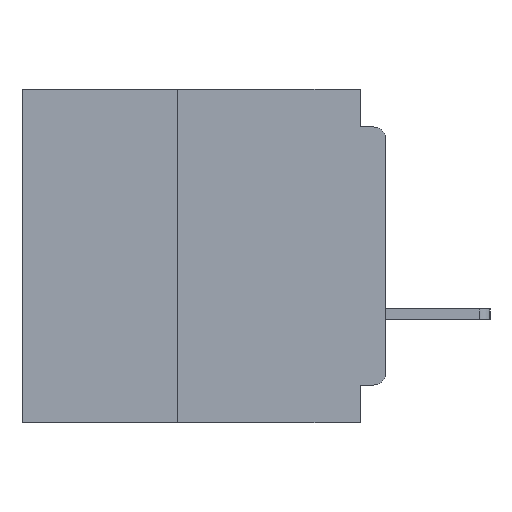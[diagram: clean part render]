
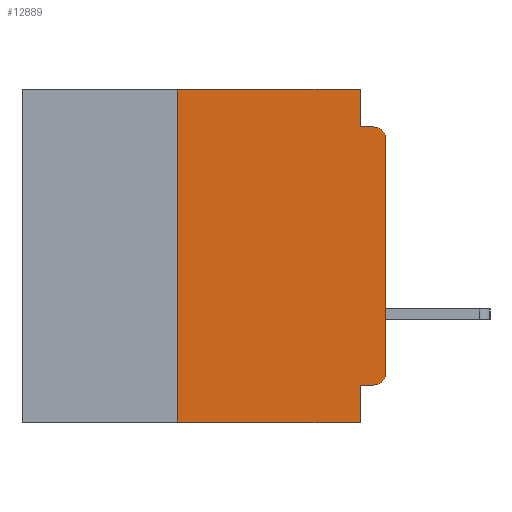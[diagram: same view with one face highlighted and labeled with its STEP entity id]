
A CAD part, left-side view. The second image highlights one B-rep face of the part: STEP entity #12889.
In plain terms, the highlighted planar face has unit normal (-1, 0, 0).
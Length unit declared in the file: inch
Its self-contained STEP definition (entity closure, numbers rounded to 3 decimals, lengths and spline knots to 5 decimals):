
#894 = VECTOR ( 'NONE', #27763, 39.37008 ) ;
#1189 = DIRECTION ( 'NONE',  ( 0., -1., 0. ) ) ;
#1572 = VECTOR ( 'NONE', #20749, 39.37008 ) ;
#1617 = CARTESIAN_POINT ( 'NONE',  ( 0., 0.031, 0. ) ) ;
#1708 = DIRECTION ( 'NONE',  ( 0., 1., 0. ) ) ;
#2461 = LINE ( 'NONE', #29116, #23068 ) ;
#2512 = VERTEX_POINT ( 'NONE', #29915 ) ;
#2609 = VECTOR ( 'NONE', #8462, 39.37008 ) ;
#3530 = CARTESIAN_POINT ( 'NONE',  ( 0., 0.015, -0.355 ) ) ;
#3698 = EDGE_CURVE ( 'NONE', #7731, #6181, #22381, .T. ) ;
#3965 = CARTESIAN_POINT ( 'NONE',  ( 0., 0., -0.045 ) ) ;
#4572 = LINE ( 'NONE', #8036, #33485 ) ;
#5168 = VERTEX_POINT ( 'NONE', #3530 ) ;
#6181 = VERTEX_POINT ( 'NONE', #33322 ) ;
#6646 = DIRECTION ( 'NONE',  ( 0., 0., 1. ) ) ;
#7092 = LINE ( 'NONE', #17834, #35963 ) ;
#7236 = CARTESIAN_POINT ( 'NONE',  ( 0., 0.25, 0. ) ) ;
#7731 = VERTEX_POINT ( 'NONE', #15136 ) ;
#8036 = CARTESIAN_POINT ( 'NONE',  ( 0., 0., 0. ) ) ;
#8047 = VERTEX_POINT ( 'NONE', #27695 ) ;
#8178 = DIRECTION ( 'NONE',  ( 1., 0., 0. ) ) ;
#8462 = DIRECTION ( 'NONE',  ( 0., -1., 0. ) ) ;
#9042 = LINE ( 'NONE', #3965, #1572 ) ;
#9081 = EDGE_CURVE ( 'NONE', #5168, #8047, #14440, .T. ) ;
#9394 = ORIENTED_EDGE ( 'NONE', *, *, #10182, .F. ) ;
#9416 = AXIS2_PLACEMENT_3D ( 'NONE', #24971, #8178, #27771 ) ;
#9592 = ORIENTED_EDGE ( 'NONE', *, *, #22513, .F. ) ;
#10182 = EDGE_CURVE ( 'NONE', #14517, #32678, #2461, .T. ) ;
#10207 = EDGE_CURVE ( 'NONE', #2512, #6181, #9042, .T. ) ;
#10853 = EDGE_CURVE ( 'NONE', #17655, #32678, #15189, .T. ) ;
#11139 = ORIENTED_EDGE ( 'NONE', *, *, #26817, .T. ) ;
#11336 = VERTEX_POINT ( 'NONE', #1617 ) ;
#12762 = CARTESIAN_POINT ( 'NONE',  ( 0., 0.015, -0.34 ) ) ;
#12889 = ADVANCED_FACE ( 'NONE', ( #33016 ), #13725, .F. ) ;
#13714 = CARTESIAN_POINT ( 'NONE',  ( 0., 0.031, 0. ) ) ;
#13725 = PLANE ( 'NONE',  #9416 ) ;
#14182 = ORIENTED_EDGE ( 'NONE', *, *, #3698, .T. ) ;
#14440 = CIRCLE ( 'NONE', #27899, 0.015 ) ;
#14517 = VERTEX_POINT ( 'NONE', #16748 ) ;
#15136 = CARTESIAN_POINT ( 'NONE',  ( 0., 0., -0.06 ) ) ;
#15189 = LINE ( 'NONE', #18070, #30052 ) ;
#15606 = DIRECTION ( 'NONE',  ( 0., 0., -1. ) ) ;
#16748 = CARTESIAN_POINT ( 'NONE',  ( 0., 0.031, -0.355 ) ) ;
#17655 = VERTEX_POINT ( 'NONE', #21581 ) ;
#17820 = ORIENTED_EDGE ( 'NONE', *, *, #25474, .F. ) ;
#17834 = CARTESIAN_POINT ( 'NONE',  ( 0., 0.25, -0.4 ) ) ;
#17948 = ORIENTED_EDGE ( 'NONE', *, *, #18972, .F. ) ;
#17984 = DIRECTION ( 'NONE',  ( 0., 0., -1. ) ) ;
#18070 = CARTESIAN_POINT ( 'NONE',  ( 0., 0.437, -0.4 ) ) ;
#18972 = EDGE_CURVE ( 'NONE', #11336, #2512, #30738, .T. ) ;
#18995 = ORIENTED_EDGE ( 'NONE', *, *, #9081, .T. ) ;
#20749 = DIRECTION ( 'NONE',  ( 0., -1., 0. ) ) ;
#20850 = EDGE_CURVE ( 'NONE', #17655, #29477, #7092, .T. ) ;
#21461 = CARTESIAN_POINT ( 'NONE',  ( 0., 0., -0.355 ) ) ;
#21581 = CARTESIAN_POINT ( 'NONE',  ( 0., 0.25, -0.4 ) ) ;
#22381 = CIRCLE ( 'NONE', #29871, 0.015 ) ;
#22513 = EDGE_CURVE ( 'NONE', #29477, #11336, #24128, .T. ) ;
#22754 = CARTESIAN_POINT ( 'NONE',  ( 0., 0.031, -0.4 ) ) ;
#23068 = VECTOR ( 'NONE', #17984, 39.37008 ) ;
#23440 = ORIENTED_EDGE ( 'NONE', *, *, #10853, .T. ) ;
#23754 = EDGE_LOOP ( 'NONE', ( #11139, #14182, #27329, #17948, #9592, #35962, #23440, #9394, #17820, #18995 ) ) ;
#24128 = LINE ( 'NONE', #25269, #2609 ) ;
#24971 = CARTESIAN_POINT ( 'NONE',  ( 0., 0.437, 0. ) ) ;
#25269 = CARTESIAN_POINT ( 'NONE',  ( 0., 0.437, 0. ) ) ;
#25474 = EDGE_CURVE ( 'NONE', #5168, #14517, #27913, .T. ) ;
#26817 = EDGE_CURVE ( 'NONE', #8047, #7731, #4572, .T. ) ;
#27329 = ORIENTED_EDGE ( 'NONE', *, *, #10207, .F. ) ;
#27629 = DIRECTION ( 'NONE',  ( 0., 0., 1. ) ) ;
#27695 = CARTESIAN_POINT ( 'NONE',  ( 0., 0., -0.34 ) ) ;
#27763 = DIRECTION ( 'NONE',  ( 0., 0., -1. ) ) ;
#27771 = DIRECTION ( 'NONE',  ( 0., 0., -1. ) ) ;
#27899 = AXIS2_PLACEMENT_3D ( 'NONE', #12762, #32338, #15606 ) ;
#27913 = LINE ( 'NONE', #21461, #34428 ) ;
#29073 = DIRECTION ( 'NONE',  ( 0., 0., -1. ) ) ;
#29116 = CARTESIAN_POINT ( 'NONE',  ( 0., 0.031, -0.4 ) ) ;
#29117 = DIRECTION ( 'NONE',  ( -1., 0., 0. ) ) ;
#29123 = CARTESIAN_POINT ( 'NONE',  ( 0., 0.015, -0.06 ) ) ;
#29477 = VERTEX_POINT ( 'NONE', #7236 ) ;
#29871 = AXIS2_PLACEMENT_3D ( 'NONE', #29123, #29117, #29073 ) ;
#29915 = CARTESIAN_POINT ( 'NONE',  ( 0., 0.031, -0.045 ) ) ;
#30052 = VECTOR ( 'NONE', #1189, 39.37008 ) ;
#30738 = LINE ( 'NONE', #13714, #894 ) ;
#32338 = DIRECTION ( 'NONE',  ( -1., 0., 0. ) ) ;
#32678 = VERTEX_POINT ( 'NONE', #22754 ) ;
#33016 = FACE_OUTER_BOUND ( 'NONE', #23754, .T. ) ;
#33322 = CARTESIAN_POINT ( 'NONE',  ( 0., 0.015, -0.045 ) ) ;
#33485 = VECTOR ( 'NONE', #27629, 39.37008 ) ;
#34428 = VECTOR ( 'NONE', #1708, 39.37008 ) ;
#35962 = ORIENTED_EDGE ( 'NONE', *, *, #20850, .F. ) ;
#35963 = VECTOR ( 'NONE', #6646, 39.37008 ) ;
